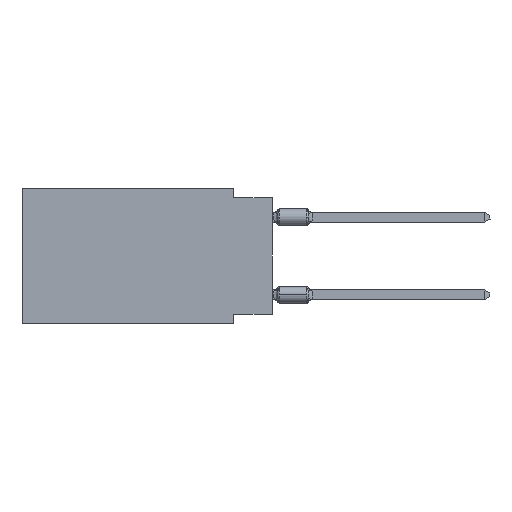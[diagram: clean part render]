
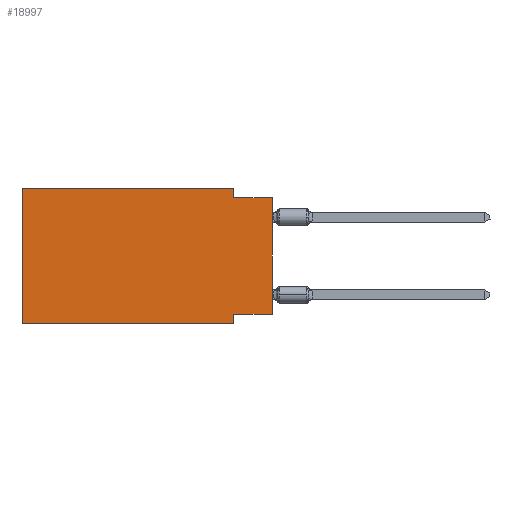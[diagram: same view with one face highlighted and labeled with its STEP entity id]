
A CAD part, left-side view. The second image highlights one B-rep face of the part: STEP entity #18997.
In plain terms, the highlighted planar face has unit normal (-1, 0, 0).
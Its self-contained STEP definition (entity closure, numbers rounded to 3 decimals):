
#75 = DIRECTION ( 'NONE',  ( 0., 0., 1. ) ) ;
#485 = DIRECTION ( 'NONE',  ( 0., -1., 0. ) ) ;
#2148 = ORIENTED_EDGE ( 'NONE', *, *, #31599, .F. ) ;
#2474 = CARTESIAN_POINT ( 'NONE',  ( 0., 2.54, -8.255 ) ) ;
#2517 = LINE ( 'NONE', #9491, #27675 ) ;
#2887 = ORIENTED_EDGE ( 'NONE', *, *, #8424, .F. ) ;
#3805 = CARTESIAN_POINT ( 'NONE',  ( 0., 0., -0.635 ) ) ;
#3896 = EDGE_CURVE ( 'NONE', #7168, #40975, #24529, .T. ) ;
#4431 = ORIENTED_EDGE ( 'NONE', *, *, #3896, .F. ) ;
#5206 = VERTEX_POINT ( 'NONE', #13147 ) ;
#5279 = DIRECTION ( 'NONE',  ( 0., 0., -1. ) ) ;
#5722 = CARTESIAN_POINT ( 'NONE',  ( 0., 16.383, -8.89 ) ) ;
#5754 = DIRECTION ( 'NONE',  ( 0., 0., 1. ) ) ;
#5951 = PLANE ( 'NONE',  #16295 ) ;
#7168 = VERTEX_POINT ( 'NONE', #37304 ) ;
#7265 = CARTESIAN_POINT ( 'NONE',  ( 0., 16.383, 0. ) ) ;
#8424 = EDGE_CURVE ( 'NONE', #42591, #38302, #2517, .T. ) ;
#9491 = CARTESIAN_POINT ( 'NONE',  ( 0., 16.383, 0. ) ) ;
#10073 = VERTEX_POINT ( 'NONE', #2474 ) ;
#10591 = CARTESIAN_POINT ( 'NONE',  ( 0., 0., -0.635 ) ) ;
#11384 = VECTOR ( 'NONE', #485, 1000. ) ;
#12400 = EDGE_CURVE ( 'NONE', #23946, #10073, #13736, .T. ) ;
#13147 = CARTESIAN_POINT ( 'NONE',  ( 0., 2.54, -8.89 ) ) ;
#13545 = EDGE_CURVE ( 'NONE', #23946, #40975, #36033, .T. ) ;
#13580 = VECTOR ( 'NONE', #75, 1000. ) ;
#13736 = LINE ( 'NONE', #20911, #36329 ) ;
#14869 = VECTOR ( 'NONE', #43629, 1000. ) ;
#16207 = CARTESIAN_POINT ( 'NONE',  ( 0., 16.383, -8.89 ) ) ;
#16295 = AXIS2_PLACEMENT_3D ( 'NONE', #19627, #39853, #5279 ) ;
#17056 = EDGE_CURVE ( 'NONE', #38302, #7168, #36140, .T. ) ;
#18978 = CARTESIAN_POINT ( 'NONE',  ( 0., 0., 0. ) ) ;
#18997 = ADVANCED_FACE ( 'NONE', ( #40303 ), #5951, .F. ) ;
#19485 = EDGE_CURVE ( 'NONE', #43620, #5206, #29454, .T. ) ;
#19627 = CARTESIAN_POINT ( 'NONE',  ( 0., 16.383, 0. ) ) ;
#20071 = LINE ( 'NONE', #7265, #13580 ) ;
#20131 = VECTOR ( 'NONE', #5754, 1000. ) ;
#20911 = CARTESIAN_POINT ( 'NONE',  ( 0., 0., -8.255 ) ) ;
#22469 = CARTESIAN_POINT ( 'NONE',  ( 0., 2.54, 0. ) ) ;
#23193 = DIRECTION ( 'NONE',  ( 0., -1., 0. ) ) ;
#23946 = VERTEX_POINT ( 'NONE', #31042 ) ;
#24529 = LINE ( 'NONE', #10591, #11384 ) ;
#26076 = ORIENTED_EDGE ( 'NONE', *, *, #12400, .F. ) ;
#26868 = CARTESIAN_POINT ( 'NONE',  ( 0., 2.54, 0. ) ) ;
#27429 = DIRECTION ( 'NONE',  ( 0., 1., 0. ) ) ;
#27675 = VECTOR ( 'NONE', #23193, 1000. ) ;
#28277 = EDGE_LOOP ( 'NONE', ( #39432, #4431, #40752, #2887, #2148, #33408, #40489, #26076 ) ) ;
#28787 = LINE ( 'NONE', #38450, #34335 ) ;
#29454 = LINE ( 'NONE', #16207, #14869 ) ;
#30593 = EDGE_CURVE ( 'NONE', #10073, #5206, #28787, .T. ) ;
#31042 = CARTESIAN_POINT ( 'NONE',  ( 0., 0., -8.255 ) ) ;
#31599 = EDGE_CURVE ( 'NONE', #43620, #42591, #20071, .T. ) ;
#32017 = VECTOR ( 'NONE', #39311, 1000. ) ;
#33408 = ORIENTED_EDGE ( 'NONE', *, *, #19485, .T. ) ;
#34335 = VECTOR ( 'NONE', #42519, 1000. ) ;
#36033 = LINE ( 'NONE', #18978, #20131 ) ;
#36140 = LINE ( 'NONE', #22469, #32017 ) ;
#36329 = VECTOR ( 'NONE', #27429, 1000. ) ;
#37304 = CARTESIAN_POINT ( 'NONE',  ( 0., 2.54, -0.635 ) ) ;
#37562 = CARTESIAN_POINT ( 'NONE',  ( 0., 16.383, 0. ) ) ;
#38302 = VERTEX_POINT ( 'NONE', #26868 ) ;
#38450 = CARTESIAN_POINT ( 'NONE',  ( 0., 2.54, -8.89 ) ) ;
#39311 = DIRECTION ( 'NONE',  ( 0., 0., -1. ) ) ;
#39432 = ORIENTED_EDGE ( 'NONE', *, *, #13545, .T. ) ;
#39853 = DIRECTION ( 'NONE',  ( 1., 0., 0. ) ) ;
#40303 = FACE_OUTER_BOUND ( 'NONE', #28277, .T. ) ;
#40489 = ORIENTED_EDGE ( 'NONE', *, *, #30593, .F. ) ;
#40752 = ORIENTED_EDGE ( 'NONE', *, *, #17056, .F. ) ;
#40975 = VERTEX_POINT ( 'NONE', #3805 ) ;
#42519 = DIRECTION ( 'NONE',  ( 0., 0., -1. ) ) ;
#42591 = VERTEX_POINT ( 'NONE', #37562 ) ;
#43620 = VERTEX_POINT ( 'NONE', #5722 ) ;
#43629 = DIRECTION ( 'NONE',  ( 0., -1., 0. ) ) ;
